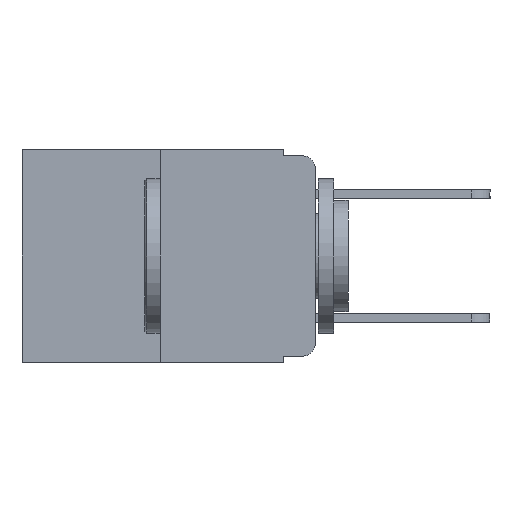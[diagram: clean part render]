
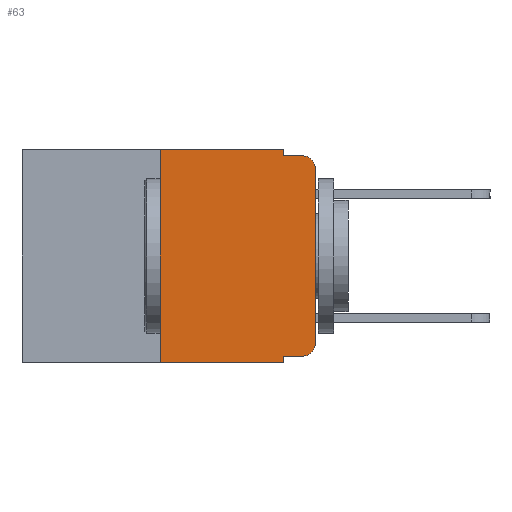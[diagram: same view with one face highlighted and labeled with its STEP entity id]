
A CAD part, left-side view. The second image highlights one B-rep face of the part: STEP entity #63.
In plain terms, the highlighted planar face has unit normal (-1, 0, 0).
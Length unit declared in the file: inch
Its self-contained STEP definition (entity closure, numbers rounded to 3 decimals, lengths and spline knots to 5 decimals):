
#63 = ADVANCED_FACE ( 'NONE', ( #1509 ), #7386, .F. ) ;
#238 = VERTEX_POINT ( 'NONE', #7738 ) ;
#277 = VECTOR ( 'NONE', #1758, 39.37008 ) ;
#339 = LINE ( 'NONE', #7829, #2795 ) ;
#416 = CARTESIAN_POINT ( 'NONE',  ( 0., 0.02, -0.03 ) ) ;
#642 = LINE ( 'NONE', #11019, #5257 ) ;
#759 = CARTESIAN_POINT ( 'NONE',  ( 0., 0.051, 0. ) ) ;
#854 = DIRECTION ( 'NONE',  ( 1., 0., 0. ) ) ;
#911 = VERTEX_POINT ( 'NONE', #4592 ) ;
#1235 = DIRECTION ( 'NONE',  ( 0., -1., 0. ) ) ;
#1261 = ORIENTED_EDGE ( 'NONE', *, *, #7286, .T. ) ;
#1415 = EDGE_CURVE ( 'NONE', #10137, #3410, #1989, .T. ) ;
#1488 = AXIS2_PLACEMENT_3D ( 'NONE', #7349, #854, #3340 ) ;
#1509 = FACE_OUTER_BOUND ( 'NONE', #3768, .T. ) ;
#1758 = DIRECTION ( 'NONE',  ( 0., -1., 0. ) ) ;
#1921 = CARTESIAN_POINT ( 'NONE',  ( 0., 0.051, -0.01 ) ) ;
#1989 = LINE ( 'NONE', #5104, #10681 ) ;
#2145 = EDGE_CURVE ( 'NONE', #10137, #2728, #642, .T. ) ;
#2308 = CIRCLE ( 'NONE', #3159, 0.02 ) ;
#2332 = DIRECTION ( 'NONE',  ( 0., -1., 0. ) ) ;
#2336 = CARTESIAN_POINT ( 'NONE',  ( 0., 0.25, 0. ) ) ;
#2728 = VERTEX_POINT ( 'NONE', #5191 ) ;
#2781 = EDGE_CURVE ( 'NONE', #4221, #238, #4786, .T. ) ;
#2795 = VECTOR ( 'NONE', #2332, 39.37008 ) ;
#2819 = ORIENTED_EDGE ( 'NONE', *, *, #1415, .T. ) ;
#2887 = VECTOR ( 'NONE', #4882, 39.37008 ) ;
#2975 = CARTESIAN_POINT ( 'NONE',  ( 0., 0.02, -0.01 ) ) ;
#3072 = VERTEX_POINT ( 'NONE', #759 ) ;
#3159 = AXIS2_PLACEMENT_3D ( 'NONE', #3531, #3519, #3575 ) ;
#3206 = ORIENTED_EDGE ( 'NONE', *, *, #9040, .F. ) ;
#3340 = DIRECTION ( 'NONE',  ( 0., 0., -1. ) ) ;
#3410 = VERTEX_POINT ( 'NONE', #5807 ) ;
#3411 = EDGE_CURVE ( 'NONE', #3072, #4640, #5371, .T. ) ;
#3519 = DIRECTION ( 'NONE',  ( -1., 0., 0. ) ) ;
#3531 = CARTESIAN_POINT ( 'NONE',  ( 0., 0.02, -0.313 ) ) ;
#3575 = DIRECTION ( 'NONE',  ( 0., 0., -1. ) ) ;
#3768 = EDGE_LOOP ( 'NONE', ( #4051, #4889, #5614, #6785, #3206, #4067, #1261, #8553, #2819, #4666 ) ) ;
#3874 = LINE ( 'NONE', #9160, #9951 ) ;
#4036 = EDGE_CURVE ( 'NONE', #4640, #8420, #9504, .T. ) ;
#4051 = ORIENTED_EDGE ( 'NONE', *, *, #5296, .T. ) ;
#4067 = ORIENTED_EDGE ( 'NONE', *, *, #2781, .F. ) ;
#4166 = AXIS2_PLACEMENT_3D ( 'NONE', #416, #4441, #4829 ) ;
#4221 = VERTEX_POINT ( 'NONE', #4336 ) ;
#4336 = CARTESIAN_POINT ( 'NONE',  ( 0., 0.25, -0.343 ) ) ;
#4441 = DIRECTION ( 'NONE',  ( -1., 0., 0. ) ) ;
#4592 = CARTESIAN_POINT ( 'NONE',  ( 0., 0., -0.03 ) ) ;
#4640 = VERTEX_POINT ( 'NONE', #7023 ) ;
#4666 = ORIENTED_EDGE ( 'NONE', *, *, #11275, .T. ) ;
#4669 = EDGE_CURVE ( 'NONE', #911, #8420, #9846, .T. ) ;
#4786 = LINE ( 'NONE', #2336, #8919 ) ;
#4829 = DIRECTION ( 'NONE',  ( 0., 0., -1. ) ) ;
#4882 = DIRECTION ( 'NONE',  ( 0., 0., -1. ) ) ;
#4889 = ORIENTED_EDGE ( 'NONE', *, *, #4669, .T. ) ;
#5104 = CARTESIAN_POINT ( 'NONE',  ( 0., 0.051, -0.333 ) ) ;
#5191 = CARTESIAN_POINT ( 'NONE',  ( 0., 0.051, -0.343 ) ) ;
#5257 = VECTOR ( 'NONE', #10988, 39.37008 ) ;
#5296 = EDGE_CURVE ( 'NONE', #5996, #911, #3874, .T. ) ;
#5371 = LINE ( 'NONE', #5710, #2887 ) ;
#5614 = ORIENTED_EDGE ( 'NONE', *, *, #4036, .F. ) ;
#5710 = CARTESIAN_POINT ( 'NONE',  ( 0., 0.051, 0. ) ) ;
#5807 = CARTESIAN_POINT ( 'NONE',  ( 0., 0.02, -0.333 ) ) ;
#5933 = LINE ( 'NONE', #9588, #9904 ) ;
#5996 = VERTEX_POINT ( 'NONE', #7717 ) ;
#6427 = CARTESIAN_POINT ( 'NONE',  ( 0., 0.051, -0.333 ) ) ;
#6785 = ORIENTED_EDGE ( 'NONE', *, *, #3411, .F. ) ;
#7023 = CARTESIAN_POINT ( 'NONE',  ( 0., 0.051, -0.01 ) ) ;
#7286 = EDGE_CURVE ( 'NONE', #4221, #2728, #339, .T. ) ;
#7349 = CARTESIAN_POINT ( 'NONE',  ( 0., 0.473, 0. ) ) ;
#7386 = PLANE ( 'NONE',  #1488 ) ;
#7457 = DIRECTION ( 'NONE',  ( 0., 0., 1. ) ) ;
#7717 = CARTESIAN_POINT ( 'NONE',  ( 0., 0., -0.313 ) ) ;
#7738 = CARTESIAN_POINT ( 'NONE',  ( 0., 0.25, 0. ) ) ;
#7829 = CARTESIAN_POINT ( 'NONE',  ( 0., 0.473, -0.343 ) ) ;
#8420 = VERTEX_POINT ( 'NONE', #2975 ) ;
#8553 = ORIENTED_EDGE ( 'NONE', *, *, #2145, .F. ) ;
#8919 = VECTOR ( 'NONE', #7457, 39.37008 ) ;
#9040 = EDGE_CURVE ( 'NONE', #238, #3072, #5933, .T. ) ;
#9160 = CARTESIAN_POINT ( 'NONE',  ( 0., 0., 0. ) ) ;
#9504 = LINE ( 'NONE', #1921, #277 ) ;
#9588 = CARTESIAN_POINT ( 'NONE',  ( 0., 0.473, 0. ) ) ;
#9612 = DIRECTION ( 'NONE',  ( 0., -1., 0. ) ) ;
#9846 = CIRCLE ( 'NONE', #4166, 0.02 ) ;
#9904 = VECTOR ( 'NONE', #9612, 39.37008 ) ;
#9951 = VECTOR ( 'NONE', #9963, 39.37008 ) ;
#9963 = DIRECTION ( 'NONE',  ( 0., 0., 1. ) ) ;
#10137 = VERTEX_POINT ( 'NONE', #6427 ) ;
#10681 = VECTOR ( 'NONE', #1235, 39.37008 ) ;
#10988 = DIRECTION ( 'NONE',  ( 0., 0., -1. ) ) ;
#11019 = CARTESIAN_POINT ( 'NONE',  ( 0., 0.051, 0. ) ) ;
#11275 = EDGE_CURVE ( 'NONE', #3410, #5996, #2308, .T. ) ;
